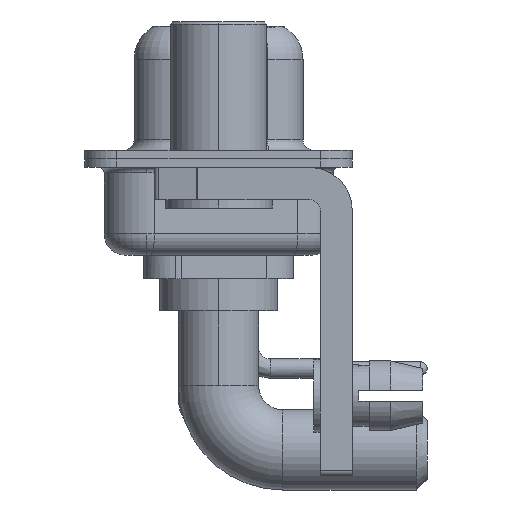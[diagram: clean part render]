
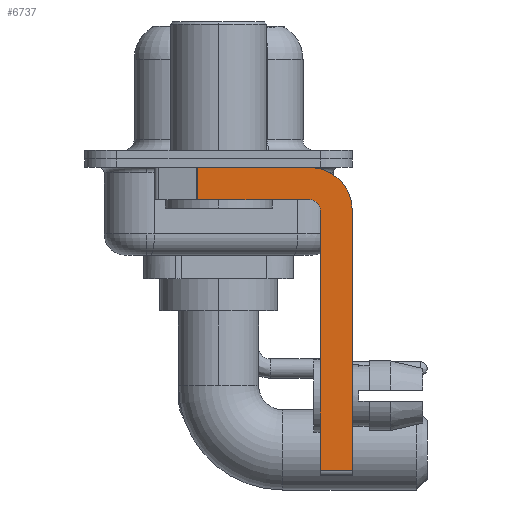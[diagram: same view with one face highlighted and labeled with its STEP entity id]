
A CAD part, left-side view. The second image highlights one B-rep face of the part: STEP entity #6737.
In plain terms, the highlighted planar face has unit normal (-1, 0, 0).
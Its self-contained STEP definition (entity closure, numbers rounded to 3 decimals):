
#993 = VERTEX_POINT ( 'NONE', #7086 ) ;
#998 = CARTESIAN_POINT ( 'NONE',  ( -2.9, -4.75, -14.8 ) ) ;
#1042 = VECTOR ( 'NONE', #21405, 1000. ) ;
#1236 = DIRECTION ( 'NONE',  ( -1., 0., 0. ) ) ;
#1673 = DIRECTION ( 'NONE',  ( 0., -1., 0. ) ) ;
#2279 = DIRECTION ( 'NONE',  ( 1., 0., 0. ) ) ;
#2540 = VERTEX_POINT ( 'NONE', #20031 ) ;
#2786 = VERTEX_POINT ( 'NONE', #8879 ) ;
#2984 = DIRECTION ( 'NONE',  ( 1., 0., 0. ) ) ;
#3360 = ORIENTED_EDGE ( 'NONE', *, *, #22648, .F. ) ;
#4262 = AXIS2_PLACEMENT_3D ( 'NONE', #13006, #1236, #4857 ) ;
#4857 = DIRECTION ( 'NONE',  ( 0., 0., 1. ) ) ;
#5056 = VECTOR ( 'NONE', #18695, 1000. ) ;
#5397 = ORIENTED_EDGE ( 'NONE', *, *, #17720, .F. ) ;
#5658 = AXIS2_PLACEMENT_3D ( 'NONE', #23563, #2984, #6353 ) ;
#5736 = CARTESIAN_POINT ( 'NONE',  ( -2.9, -6.25, -2.4 ) ) ;
#6077 = VERTEX_POINT ( 'NONE', #16904 ) ;
#6353 = DIRECTION ( 'NONE',  ( 0., 0., -1. ) ) ;
#6737 = ADVANCED_FACE ( 'NONE', ( #7771 ), #15675, .F. ) ;
#6804 = CARTESIAN_POINT ( 'NONE',  ( -2.9, -4.25, -1.9 ) ) ;
#7086 = CARTESIAN_POINT ( 'NONE',  ( -2.9, -4.75, -2.4 ) ) ;
#7399 = DIRECTION ( 'NONE',  ( 0., 0., -1. ) ) ;
#7771 = FACE_OUTER_BOUND ( 'NONE', #8822, .T. ) ;
#7873 = AXIS2_PLACEMENT_3D ( 'NONE', #8594, #2279, #10535 ) ;
#8201 = CARTESIAN_POINT ( 'NONE',  ( -2.9, 0.978, -1.9 ) ) ;
#8558 = EDGE_CURVE ( 'NONE', #6077, #2786, #21378, .T. ) ;
#8594 = CARTESIAN_POINT ( 'NONE',  ( -2.9, -4.25, -2.4 ) ) ;
#8822 = EDGE_LOOP ( 'NONE', ( #23931, #24087, #5397, #3360, #20911, #9429, #17039, #14828 ) ) ;
#8879 = CARTESIAN_POINT ( 'NONE',  ( -2.9, -6.25, -14.55 ) ) ;
#9360 = CARTESIAN_POINT ( 'NONE',  ( -2.9, -4.25, -14.55 ) ) ;
#9429 = ORIENTED_EDGE ( 'NONE', *, *, #9708, .T. ) ;
#9708 = EDGE_CURVE ( 'NONE', #2540, #2786, #19195, .T. ) ;
#10065 = CIRCLE ( 'NONE', #4262, 0.5 ) ;
#10246 = VERTEX_POINT ( 'NONE', #18793 ) ;
#10535 = DIRECTION ( 'NONE',  ( 0., 0., -1. ) ) ;
#10676 = CARTESIAN_POINT ( 'NONE',  ( -2.9, 0.978, -1.9 ) ) ;
#10826 = DIRECTION ( 'NONE',  ( 0., 0., 1. ) ) ;
#12660 = EDGE_CURVE ( 'NONE', #10246, #6077, #14512, .T. ) ;
#13006 = CARTESIAN_POINT ( 'NONE',  ( -2.9, -4.25, -2.4 ) ) ;
#13647 = CARTESIAN_POINT ( 'NONE',  ( -2.9, -4.25, -1.9 ) ) ;
#14512 = CIRCLE ( 'NONE', #7873, 2. ) ;
#14828 = ORIENTED_EDGE ( 'NONE', *, *, #12660, .F. ) ;
#15423 = VECTOR ( 'NONE', #1673, 1000. ) ;
#15675 = PLANE ( 'NONE',  #5658 ) ;
#15763 = CARTESIAN_POINT ( 'NONE',  ( -2.9, 3., -0.4 ) ) ;
#15853 = LINE ( 'NONE', #13647, #1042 ) ;
#15922 = VERTEX_POINT ( 'NONE', #6804 ) ;
#16904 = CARTESIAN_POINT ( 'NONE',  ( -2.9, -6.25, -2.4 ) ) ;
#17039 = ORIENTED_EDGE ( 'NONE', *, *, #8558, .F. ) ;
#17131 = DIRECTION ( 'NONE',  ( 0., -1., 0. ) ) ;
#17720 = EDGE_CURVE ( 'NONE', #15922, #22972, #15853, .T. ) ;
#18695 = DIRECTION ( 'NONE',  ( 0., 0., -1. ) ) ;
#18793 = CARTESIAN_POINT ( 'NONE',  ( -2.9, -4.25, -0.4 ) ) ;
#19195 = LINE ( 'NONE', #9360, #21470 ) ;
#19715 = VERTEX_POINT ( 'NONE', #23716 ) ;
#20031 = CARTESIAN_POINT ( 'NONE',  ( -2.9, -4.75, -14.55 ) ) ;
#20215 = EDGE_CURVE ( 'NONE', #19715, #22972, #22948, .T. ) ;
#20602 = VECTOR ( 'NONE', #7399, 1000. ) ;
#20748 = EDGE_CURVE ( 'NONE', #19715, #10246, #21577, .T. ) ;
#20911 = ORIENTED_EDGE ( 'NONE', *, *, #24845, .F. ) ;
#21378 = LINE ( 'NONE', #5736, #20602 ) ;
#21405 = DIRECTION ( 'NONE',  ( 0., 1., 0. ) ) ;
#21470 = VECTOR ( 'NONE', #17131, 1000. ) ;
#21577 = LINE ( 'NONE', #15763, #15423 ) ;
#22648 = EDGE_CURVE ( 'NONE', #993, #15922, #10065, .T. ) ;
#22948 = LINE ( 'NONE', #10676, #5056 ) ;
#22972 = VERTEX_POINT ( 'NONE', #8201 ) ;
#23563 = CARTESIAN_POINT ( 'NONE',  ( -2.9, -4.25, -2.4 ) ) ;
#23716 = CARTESIAN_POINT ( 'NONE',  ( -2.9, 0.978, -0.4 ) ) ;
#23804 = VECTOR ( 'NONE', #10826, 1000. ) ;
#23931 = ORIENTED_EDGE ( 'NONE', *, *, #20748, .F. ) ;
#24087 = ORIENTED_EDGE ( 'NONE', *, *, #20215, .T. ) ;
#24409 = LINE ( 'NONE', #998, #23804 ) ;
#24845 = EDGE_CURVE ( 'NONE', #2540, #993, #24409, .T. ) ;
